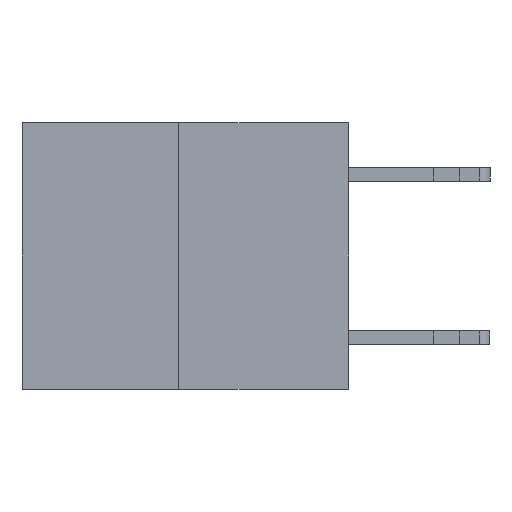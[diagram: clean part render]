
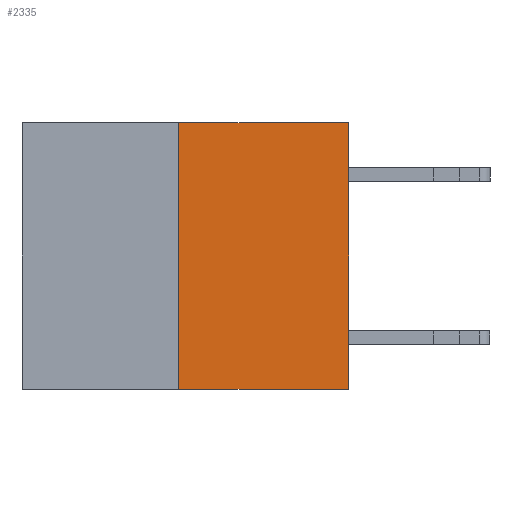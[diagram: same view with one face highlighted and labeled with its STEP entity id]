
A CAD part, left-side view. The second image highlights one B-rep face of the part: STEP entity #2335.
In plain terms, the highlighted planar face has unit normal (-1, 0, 0).
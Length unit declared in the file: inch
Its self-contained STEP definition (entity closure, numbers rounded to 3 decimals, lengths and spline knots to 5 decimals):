
#67 = VECTOR ( 'NONE', #5895, 39.37008 ) ;
#889 = ORIENTED_EDGE ( 'NONE', *, *, #8960, .F. ) ;
#949 = FACE_OUTER_BOUND ( 'NONE', #3207, .T. ) ;
#1052 = LINE ( 'NONE', #4369, #7403 ) ;
#1276 = VERTEX_POINT ( 'NONE', #16742 ) ;
#1394 = DIRECTION ( 'NONE',  ( 0., -1., 0. ) ) ;
#1445 = LINE ( 'NONE', #16438, #10910 ) ;
#1756 = DIRECTION ( 'NONE',  ( 0., 0., -1. ) ) ;
#1785 = ORIENTED_EDGE ( 'NONE', *, *, #11315, .T. ) ;
#2335 = ADVANCED_FACE ( 'NONE', ( #949 ), #15316, .F. ) ;
#3207 = EDGE_LOOP ( 'NONE', ( #889, #10351, #1785, #14516 ) ) ;
#4369 = CARTESIAN_POINT ( 'NONE',  ( 0., 0., 0. ) ) ;
#4503 = CARTESIAN_POINT ( 'NONE',  ( 0., 0.6, -0.49 ) ) ;
#5477 = EDGE_CURVE ( 'NONE', #5928, #1276, #6123, .T. ) ;
#5658 = EDGE_CURVE ( 'NONE', #13500, #8080, #1445, .T. ) ;
#5895 = DIRECTION ( 'NONE',  ( 0., 0., 1. ) ) ;
#5928 = VERTEX_POINT ( 'NONE', #10164 ) ;
#5938 = DIRECTION ( 'NONE',  ( 1., 0., 0. ) ) ;
#6075 = CARTESIAN_POINT ( 'NONE',  ( 0., 0.312, -0.49 ) ) ;
#6123 = LINE ( 'NONE', #4503, #12845 ) ;
#7119 = DIRECTION ( 'NONE',  ( 0., -1., 0. ) ) ;
#7403 = VECTOR ( 'NONE', #11183, 39.37008 ) ;
#8080 = VERTEX_POINT ( 'NONE', #11718 ) ;
#8960 = EDGE_CURVE ( 'NONE', #5928, #13500, #12080, .T. ) ;
#10164 = CARTESIAN_POINT ( 'NONE',  ( 0., 0.312, -0.49 ) ) ;
#10351 = ORIENTED_EDGE ( 'NONE', *, *, #5477, .T. ) ;
#10910 = VECTOR ( 'NONE', #1394, 39.37008 ) ;
#11183 = DIRECTION ( 'NONE',  ( 0., 0., 1. ) ) ;
#11315 = EDGE_CURVE ( 'NONE', #1276, #8080, #1052, .T. ) ;
#11718 = CARTESIAN_POINT ( 'NONE',  ( 0., 0., 0. ) ) ;
#12080 = LINE ( 'NONE', #6075, #67 ) ;
#12421 = CARTESIAN_POINT ( 'NONE',  ( 0., 0.6, 0. ) ) ;
#12845 = VECTOR ( 'NONE', #7119, 39.37008 ) ;
#13500 = VERTEX_POINT ( 'NONE', #14148 ) ;
#14148 = CARTESIAN_POINT ( 'NONE',  ( 0., 0.312, 0. ) ) ;
#14516 = ORIENTED_EDGE ( 'NONE', *, *, #5658, .F. ) ;
#15316 = PLANE ( 'NONE',  #16372 ) ;
#16372 = AXIS2_PLACEMENT_3D ( 'NONE', #12421, #5938, #1756 ) ;
#16438 = CARTESIAN_POINT ( 'NONE',  ( 0., 0.6, 0. ) ) ;
#16742 = CARTESIAN_POINT ( 'NONE',  ( 0., 0., -0.49 ) ) ;
